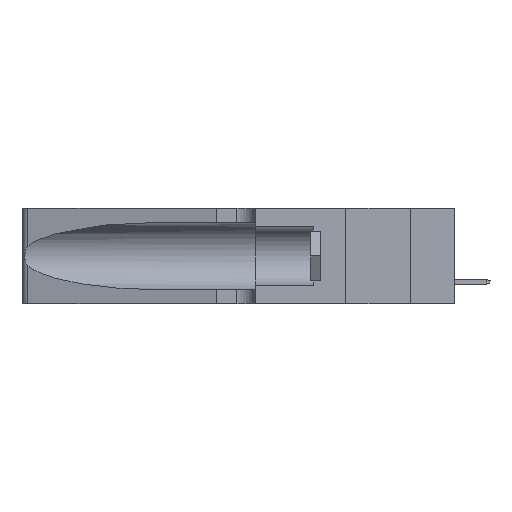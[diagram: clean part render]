
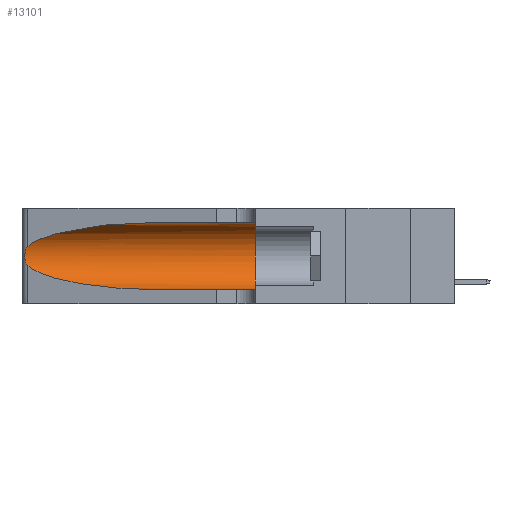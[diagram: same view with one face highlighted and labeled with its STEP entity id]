
A CAD part, left-side view. The second image highlights one B-rep face of the part: STEP entity #13101.
In plain terms, the highlighted cylindrical face has radius 3.308 mm (diameter 6.617 mm), a partial arc.
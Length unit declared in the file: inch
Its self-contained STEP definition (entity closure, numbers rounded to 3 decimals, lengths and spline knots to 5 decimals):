
#362 = CARTESIAN_POINT ( 'NONE',  ( 0.25487, 1.22718, 0.22369 ) ) ;
#626 = ORIENTED_EDGE ( 'NONE', *, *, #11882, .F. ) ;
#1144 = CARTESIAN_POINT ( 'NONE',  ( 0.26017, 1.23833, 0.17102 ) ) ;
#1808 = EDGE_CURVE ( 'NONE', #4630, #6873, #13005, .T. ) ;
#2440 = CYLINDRICAL_SURFACE ( 'NONE', #18251, 0.13025 ) ;
#2654 = DIRECTION ( 'NONE',  ( 0., 0., -1. ) ) ;
#2987 = DIRECTION ( 'NONE',  ( 0., -1., 0. ) ) ;
#3990 = CARTESIAN_POINT ( 'NONE',  ( 0.25487, 1.22718, 0.22369 ) ) ;
#4630 = VERTEX_POINT ( 'NONE', #3990 ) ;
#6873 = VERTEX_POINT ( 'NONE', #11755 ) ;
#7260 =( BOUNDED_CURVE ( )  B_SPLINE_CURVE ( 3, ( #17219, #37494, #30741, #362 ),
 .UNSPECIFIED., .F., .F. ) 
 B_SPLINE_CURVE_WITH_KNOTS ( ( 4, 4 ),
 ( 1.5708, 2.84003 ),
 .UNSPECIFIED. ) 
 CURVE ( )  GEOMETRIC_REPRESENTATION_ITEM ( )  RATIONAL_B_SPLINE_CURVE ( ( 1., 0.87, 0.87, 1. ) ) 
 REPRESENTATION_ITEM ( '' )  );
#7678 = EDGE_CURVE ( 'NONE', #37097, #4630, #7260, .T. ) ;
#8525 = DIRECTION ( 'NONE',  ( 0., 0., 1. ) ) ;
#10136 = CARTESIAN_POINT ( 'NONE',  ( 0.25854, 1.2359, 0.20912 ) ) ;
#11481 = CARTESIAN_POINT ( 'NONE',  ( 0.25789, 1.23486, 0.15765 ) ) ;
#11755 = CARTESIAN_POINT ( 'NONE',  ( 0.25487, 1.22718, 0.14631 ) ) ;
#11882 = EDGE_CURVE ( 'NONE', #37097, #30507, #26318, .T. ) ;
#12016 = ORIENTED_EDGE ( 'NONE', *, *, #29808, .T. ) ;
#12554 = DIRECTION ( 'NONE',  ( 0., -1., 0. ) ) ;
#13005 = B_SPLINE_CURVE_WITH_KNOTS ( 'NONE', 3,
 ( #20040, #16660, #40976, #30409, #10136, #20479, #42109, #21378, #1144, #32189, #11481, #14859, #35112, #28152 ),
 .UNSPECIFIED., .F., .F.,
 ( 4, 2, 2, 2, 2, 2, 4 ),
 ( 0., 0.00027, 0.00053, 0.00107, 0.0016, 0.00187, 0.00214 ),
 .UNSPECIFIED. ) ;
#13101 = ADVANCED_FACE ( 'NONE', ( #39797 ), #2440, .F. ) ;
#14221 = EDGE_CURVE ( 'NONE', #6873, #17908, #18178, .T. ) ;
#14319 = ORIENTED_EDGE ( 'NONE', *, *, #36328, .F. ) ;
#14578 = VECTOR ( 'NONE', #2987, 39.37008 ) ;
#14634 = AXIS2_PLACEMENT_3D ( 'NONE', #39350, #43782, #8525 ) ;
#14859 = CARTESIAN_POINT ( 'NONE',  ( 0.25639, 1.23186, 0.15144 ) ) ;
#14886 = CARTESIAN_POINT ( 'NONE',  ( 0.25487, 1.22718, 0.14631 ) ) ;
#16660 = CARTESIAN_POINT ( 'NONE',  ( 0.25555, 1.22994, 0.2215 ) ) ;
#17219 = CARTESIAN_POINT ( 'NONE',  ( 0.1305, 0.72297, 0.31525 ) ) ;
#17908 = VERTEX_POINT ( 'NONE', #22957 ) ;
#18178 =( BOUNDED_CURVE ( )  B_SPLINE_CURVE ( 3, ( #14886, #21860, #35365, #42364 ),
 .UNSPECIFIED., .F., .F. ) 
 B_SPLINE_CURVE_WITH_KNOTS ( ( 4, 4 ),
 ( 3.44316, 4.71239 ),
 .UNSPECIFIED. ) 
 CURVE ( )  GEOMETRIC_REPRESENTATION_ITEM ( )  RATIONAL_B_SPLINE_CURVE ( ( 1., 0.87, 0.87, 1. ) ) 
 REPRESENTATION_ITEM ( '' )  );
#18251 = AXIS2_PLACEMENT_3D ( 'NONE', #26285, #12554, #2654 ) ;
#20040 = CARTESIAN_POINT ( 'NONE',  ( 0.25487, 1.22718, 0.22369 ) ) ;
#20293 = VECTOR ( 'NONE', #33061, 39.37008 ) ;
#20479 = CARTESIAN_POINT ( 'NONE',  ( 0.26018, 1.23835, 0.19895 ) ) ;
#21378 = CARTESIAN_POINT ( 'NONE',  ( 0.26075, 1.23896, 0.178 ) ) ;
#21860 = CARTESIAN_POINT ( 'NONE',  ( 0.2373, 1.15595, 0.08982 ) ) ;
#22601 = ORIENTED_EDGE ( 'NONE', *, *, #1808, .T. ) ;
#22712 = CARTESIAN_POINT ( 'NONE',  ( 0.1305, 1.61858, 0.31525 ) ) ;
#22957 = CARTESIAN_POINT ( 'NONE',  ( 0.1305, 0.72297, 0.05475 ) ) ;
#26052 = ORIENTED_EDGE ( 'NONE', *, *, #14221, .T. ) ;
#26285 = CARTESIAN_POINT ( 'NONE',  ( 0.1305, 1.61858, 0.185 ) ) ;
#26318 = LINE ( 'NONE', #22712, #20293 ) ;
#27525 = LINE ( 'NONE', #31333, #14578 ) ;
#27690 = CARTESIAN_POINT ( 'NONE',  ( 0.1305, 0.35, 0.05475 ) ) ;
#28152 = CARTESIAN_POINT ( 'NONE',  ( 0.25487, 1.22718, 0.14631 ) ) ;
#29808 = EDGE_CURVE ( 'NONE', #17908, #40133, #27525, .T. ) ;
#30409 = CARTESIAN_POINT ( 'NONE',  ( 0.25787, 1.23484, 0.2124 ) ) ;
#30507 = VERTEX_POINT ( 'NONE', #40415 ) ;
#30741 = CARTESIAN_POINT ( 'NONE',  ( 0.2373, 1.15595, 0.28018 ) ) ;
#31333 = CARTESIAN_POINT ( 'NONE',  ( 0.1305, 1.61858, 0.05475 ) ) ;
#32189 = CARTESIAN_POINT ( 'NONE',  ( 0.25856, 1.23593, 0.16098 ) ) ;
#33061 = DIRECTION ( 'NONE',  ( 0., -1., 0. ) ) ;
#34011 = CIRCLE ( 'NONE', #14634, 0.13025 ) ;
#35112 = CARTESIAN_POINT ( 'NONE',  ( 0.25555, 1.22993, 0.14849 ) ) ;
#35365 = CARTESIAN_POINT ( 'NONE',  ( 0.18966, 0.96281, 0.05475 ) ) ;
#35911 = EDGE_LOOP ( 'NONE', ( #40711, #22601, #26052, #12016, #14319, #626 ) ) ;
#36328 = EDGE_CURVE ( 'NONE', #30507, #40133, #34011, .T. ) ;
#37097 = VERTEX_POINT ( 'NONE', #37795 ) ;
#37494 = CARTESIAN_POINT ( 'NONE',  ( 0.18966, 0.96281, 0.31525 ) ) ;
#37795 = CARTESIAN_POINT ( 'NONE',  ( 0.1305, 0.72297, 0.31525 ) ) ;
#39350 = CARTESIAN_POINT ( 'NONE',  ( 0.1305, 0.35, 0.185 ) ) ;
#39797 = FACE_OUTER_BOUND ( 'NONE', #35911, .T. ) ;
#40133 = VERTEX_POINT ( 'NONE', #27690 ) ;
#40415 = CARTESIAN_POINT ( 'NONE',  ( 0.1305, 0.35, 0.31525 ) ) ;
#40711 = ORIENTED_EDGE ( 'NONE', *, *, #7678, .T. ) ;
#40976 = CARTESIAN_POINT ( 'NONE',  ( 0.25639, 1.23184, 0.21858 ) ) ;
#42109 = CARTESIAN_POINT ( 'NONE',  ( 0.26075, 1.23896, 0.19203 ) ) ;
#42364 = CARTESIAN_POINT ( 'NONE',  ( 0.1305, 0.72297, 0.05475 ) ) ;
#43782 = DIRECTION ( 'NONE',  ( 0., 1., 0. ) ) ;
